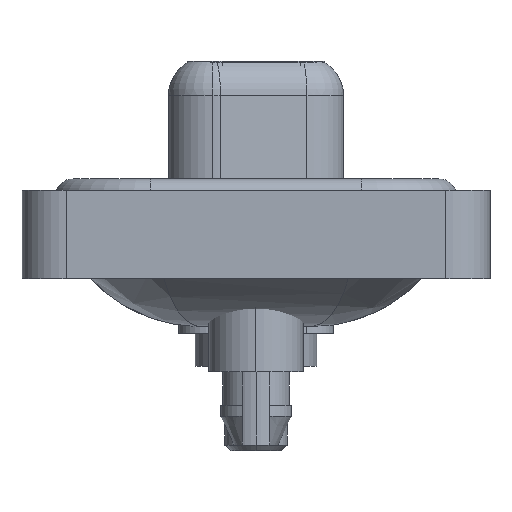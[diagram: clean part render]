
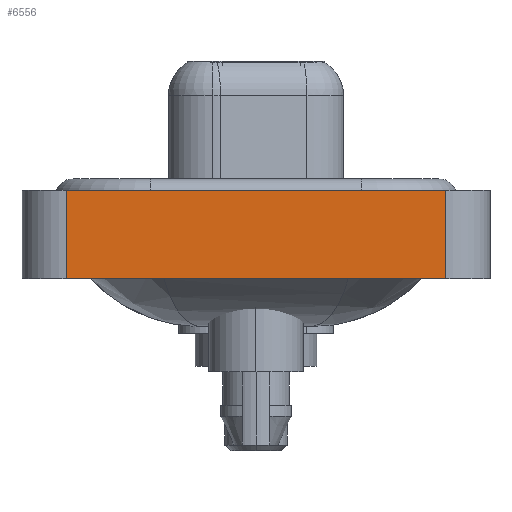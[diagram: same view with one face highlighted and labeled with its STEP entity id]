
A CAD part, left-side view. The second image highlights one B-rep face of the part: STEP entity #6556.
In plain terms, the highlighted planar face has unit normal (-1, 0, 0).
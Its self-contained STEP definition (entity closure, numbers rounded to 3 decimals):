
#55 = VERTEX_POINT ( 'NONE', #14509 ) ;
#167 = ORIENTED_EDGE ( 'NONE', *, *, #11544, .T. ) ;
#812 = DIRECTION ( 'NONE',  ( 0., 0., 1. ) ) ;
#1432 = CARTESIAN_POINT ( 'NONE',  ( -7.25, -8.55, 0.4 ) ) ;
#2443 = VERTEX_POINT ( 'NONE', #1432 ) ;
#2535 = EDGE_CURVE ( 'NONE', #10773, #15193, #8401, .T. ) ;
#3309 = FACE_OUTER_BOUND ( 'NONE', #9791, .T. ) ;
#4031 = VECTOR ( 'NONE', #9931, 1000. ) ;
#5425 = DIRECTION ( 'NONE',  ( 0., 0., 1. ) ) ;
#5985 = VECTOR ( 'NONE', #5425, 1000. ) ;
#6298 = CARTESIAN_POINT ( 'NONE',  ( -7.25, 8.55, 0.4 ) ) ;
#6454 = ORIENTED_EDGE ( 'NONE', *, *, #2535, .F. ) ;
#6515 = LINE ( 'NONE', #11714, #14200 ) ;
#6556 = ADVANCED_FACE ( 'NONE', ( #3309 ), #13537, .T. ) ;
#6742 = EDGE_CURVE ( 'NONE', #10773, #55, #6515, .T. ) ;
#6977 = AXIS2_PLACEMENT_3D ( 'NONE', #7171, #12282, #812 ) ;
#7171 = CARTESIAN_POINT ( 'NONE',  ( -7.25, -8.55, -3.6 ) ) ;
#7206 = DIRECTION ( 'NONE',  ( 0., 0., 1. ) ) ;
#7895 = ORIENTED_EDGE ( 'NONE', *, *, #6742, .T. ) ;
#8001 = CARTESIAN_POINT ( 'NONE',  ( -7.25, 8.55, -3.6 ) ) ;
#8401 = LINE ( 'NONE', #14589, #10159 ) ;
#9791 = EDGE_LOOP ( 'NONE', ( #167, #14338, #6454, #7895 ) ) ;
#9931 = DIRECTION ( 'NONE',  ( 0., -1., 0. ) ) ;
#10159 = VECTOR ( 'NONE', #7206, 1000. ) ;
#10773 = VERTEX_POINT ( 'NONE', #8001 ) ;
#11009 = CARTESIAN_POINT ( 'NONE',  ( -7.25, -8.55, 0.4 ) ) ;
#11544 = EDGE_CURVE ( 'NONE', #55, #2443, #11965, .T. ) ;
#11714 = CARTESIAN_POINT ( 'NONE',  ( -7.25, -8.55, -3.6 ) ) ;
#11965 = LINE ( 'NONE', #12047, #5985 ) ;
#12047 = CARTESIAN_POINT ( 'NONE',  ( -7.25, -8.55, -3.6 ) ) ;
#12282 = DIRECTION ( 'NONE',  ( -1., 0., 0. ) ) ;
#12348 = LINE ( 'NONE', #11009, #4031 ) ;
#13537 = PLANE ( 'NONE',  #6977 ) ;
#13822 = EDGE_CURVE ( 'NONE', #15193, #2443, #12348, .T. ) ;
#14044 = DIRECTION ( 'NONE',  ( 0., -1., 0. ) ) ;
#14200 = VECTOR ( 'NONE', #14044, 1000. ) ;
#14338 = ORIENTED_EDGE ( 'NONE', *, *, #13822, .F. ) ;
#14509 = CARTESIAN_POINT ( 'NONE',  ( -7.25, -8.55, -3.6 ) ) ;
#14589 = CARTESIAN_POINT ( 'NONE',  ( -7.25, 8.55, -3.6 ) ) ;
#15193 = VERTEX_POINT ( 'NONE', #6298 ) ;
